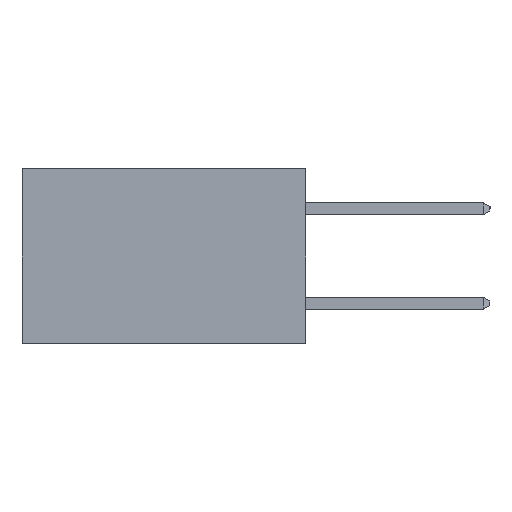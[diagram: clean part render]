
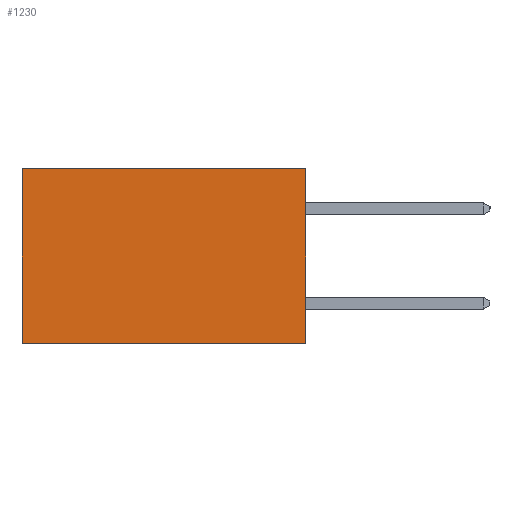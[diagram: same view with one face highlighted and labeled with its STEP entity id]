
A CAD part, left-side view. The second image highlights one B-rep face of the part: STEP entity #1230.
In plain terms, the highlighted planar face has unit normal (-1, 0, 0).
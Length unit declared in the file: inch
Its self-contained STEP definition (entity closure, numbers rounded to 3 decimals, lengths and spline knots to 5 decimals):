
#568 = DIRECTION ( 'NONE',  ( 0., 0., -1. ) ) ;
#615 = VECTOR ( 'NONE', #2376, 39.37008 ) ;
#1230 = ADVANCED_FACE ( 'NONE', ( #10422 ), #5411, .F. ) ;
#1441 = EDGE_CURVE ( 'NONE', #9236, #7255, #7600, .T. ) ;
#1535 = VECTOR ( 'NONE', #10711, 39.37008 ) ;
#1593 = DIRECTION ( 'NONE',  ( 0., 1., 0. ) ) ;
#1974 = CARTESIAN_POINT ( 'NONE',  ( 0.2615, 0., -0.37 ) ) ;
#2183 = ORIENTED_EDGE ( 'NONE', *, *, #3927, .F. ) ;
#2376 = DIRECTION ( 'NONE',  ( 0., 1., 0. ) ) ;
#2585 = VECTOR ( 'NONE', #1593, 39.37008 ) ;
#3186 = LINE ( 'NONE', #10789, #2585 ) ;
#3219 = VERTEX_POINT ( 'NONE', #5570 ) ;
#3248 = CARTESIAN_POINT ( 'NONE',  ( 0.2615, 0., 0. ) ) ;
#3823 = EDGE_LOOP ( 'NONE', ( #8455, #2183, #7492, #10649 ) ) ;
#3855 = CARTESIAN_POINT ( 'NONE',  ( 0.2615, 0.6, 0. ) ) ;
#3877 = LINE ( 'NONE', #4848, #1535 ) ;
#3926 = CARTESIAN_POINT ( 'NONE',  ( 0.2615, 0., -0.37 ) ) ;
#3927 = EDGE_CURVE ( 'NONE', #5424, #3219, #3186, .T. ) ;
#4087 = DIRECTION ( 'NONE',  ( 0., 0., -1. ) ) ;
#4307 = CARTESIAN_POINT ( 'NONE',  ( 0.2615, 0., -0.37 ) ) ;
#4445 = CARTESIAN_POINT ( 'NONE',  ( 0.2615, 0., 0. ) ) ;
#4848 = CARTESIAN_POINT ( 'NONE',  ( 0.2615, 0.6, -0.37 ) ) ;
#5411 = PLANE ( 'NONE',  #9727 ) ;
#5424 = VERTEX_POINT ( 'NONE', #1974 ) ;
#5570 = CARTESIAN_POINT ( 'NONE',  ( 0.2615, 0.6, -0.37 ) ) ;
#5790 = LINE ( 'NONE', #4307, #10279 ) ;
#7255 = VERTEX_POINT ( 'NONE', #3855 ) ;
#7492 = ORIENTED_EDGE ( 'NONE', *, *, #8159, .F. ) ;
#7600 = LINE ( 'NONE', #3248, #615 ) ;
#7967 = EDGE_CURVE ( 'NONE', #7255, #3219, #3877, .T. ) ;
#8102 = DIRECTION ( 'NONE',  ( 1., 0., 0. ) ) ;
#8159 = EDGE_CURVE ( 'NONE', #9236, #5424, #5790, .T. ) ;
#8455 = ORIENTED_EDGE ( 'NONE', *, *, #7967, .T. ) ;
#9236 = VERTEX_POINT ( 'NONE', #4445 ) ;
#9727 = AXIS2_PLACEMENT_3D ( 'NONE', #3926, #8102, #568 ) ;
#10279 = VECTOR ( 'NONE', #4087, 39.37008 ) ;
#10422 = FACE_OUTER_BOUND ( 'NONE', #3823, .T. ) ;
#10649 = ORIENTED_EDGE ( 'NONE', *, *, #1441, .T. ) ;
#10711 = DIRECTION ( 'NONE',  ( 0., 0., -1. ) ) ;
#10789 = CARTESIAN_POINT ( 'NONE',  ( 0.2615, 0., -0.37 ) ) ;
